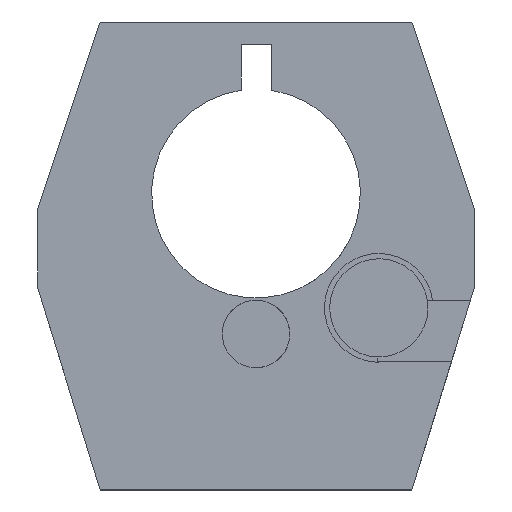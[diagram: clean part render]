
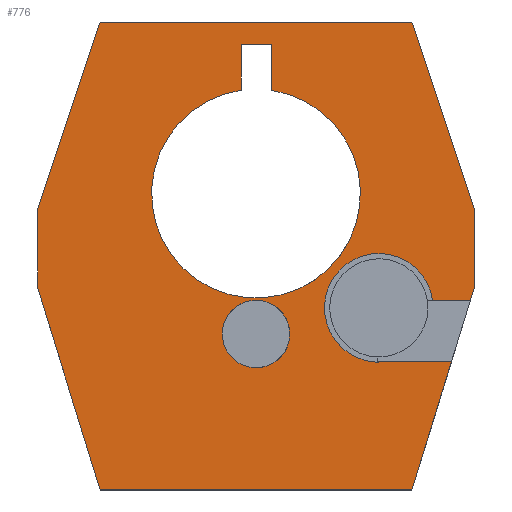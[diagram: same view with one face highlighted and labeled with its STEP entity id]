
A CAD part, front view. The second image highlights one B-rep face of the part: STEP entity #776.
In plain terms, the highlighted planar face has unit normal (0, -1, 0).
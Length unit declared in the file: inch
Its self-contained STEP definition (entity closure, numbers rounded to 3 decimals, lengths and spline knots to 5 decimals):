
#29=FACE_BOUND('',#122,.T.);
#30=FACE_BOUND('',#123,.T.);
#40=CIRCLE('',#836,0.10827);
#41=CIRCLE('',#837,0.10827);
#43=CIRCLE('',#844,0.17421);
#44=CIRCLE('',#846,0.33465);
#77=FACE_OUTER_BOUND('',#121,.T.);
#121=EDGE_LOOP('',(#650,#651,#652,#653,#654,#655,#656,#657,#658,#659,#660,
#661,#662,#663,#664,#665));
#122=EDGE_LOOP('',(#666,#667,#668,#669));
#123=EDGE_LOOP('',(#670,#671));
#162=LINE('',#1124,#253);
#166=LINE('',#1132,#257);
#168=LINE('',#1140,#259);
#174=LINE('',#1152,#265);
#177=LINE('',#1157,#268);
#180=LINE('',#1163,#271);
#184=LINE('',#1172,#275);
#187=LINE('',#1177,#278);
#194=LINE('',#1193,#285);
#203=LINE('',#1226,#294);
#206=LINE('',#1230,#297);
#210=LINE('',#1284,#301);
#212=LINE('',#1289,#303);
#213=LINE('',#1291,#304);
#214=LINE('',#1293,#305);
#215=LINE('',#1295,#306);
#216=LINE('',#1296,#307);
#217=LINE('',#1299,#308);
#253=VECTOR('',#906,0.3937);
#257=VECTOR('',#910,0.3937);
#259=VECTOR('',#918,0.3937);
#265=VECTOR('',#926,0.3937);
#268=VECTOR('',#931,0.3937);
#271=VECTOR('',#936,0.3937);
#275=VECTOR('',#944,0.3937);
#278=VECTOR('',#949,0.3937);
#285=VECTOR('',#962,0.3937);
#294=VECTOR('',#997,0.3937);
#297=VECTOR('',#1002,0.3937);
#301=VECTOR('',#1022,0.3937);
#303=VECTOR('',#1030,0.3937);
#304=VECTOR('',#1031,0.3937);
#305=VECTOR('',#1032,0.3937);
#306=VECTOR('',#1033,0.3937);
#307=VECTOR('',#1034,0.3937);
#308=VECTOR('',#1037,0.3937);
#337=VERTEX_POINT('',#1121);
#338=VERTEX_POINT('',#1123);
#341=VERTEX_POINT('',#1129);
#342=VERTEX_POINT('',#1131);
#345=VERTEX_POINT('',#1139);
#349=VERTEX_POINT('',#1149);
#350=VERTEX_POINT('',#1151);
#351=VERTEX_POINT('',#1155);
#353=VERTEX_POINT('',#1161);
#355=VERTEX_POINT('',#1169);
#356=VERTEX_POINT('',#1171);
#357=VERTEX_POINT('',#1175);
#363=VERTEX_POINT('',#1191);
#373=VERTEX_POINT('',#1223);
#374=VERTEX_POINT('',#1225);
#375=VERTEX_POINT('',#1232);
#376=VERTEX_POINT('',#1233);
#380=VERTEX_POINT('',#1283);
#381=VERTEX_POINT('',#1290);
#382=VERTEX_POINT('',#1292);
#383=VERTEX_POINT('',#1294);
#384=VERTEX_POINT('',#1297);
#416=EDGE_CURVE('',#338,#337,#162,.T.);
#420=EDGE_CURVE('',#342,#341,#166,.T.);
#424=EDGE_CURVE('',#345,#342,#168,.T.);
#430=EDGE_CURVE('',#350,#349,#174,.T.);
#433=EDGE_CURVE('',#349,#351,#177,.T.);
#436=EDGE_CURVE('',#337,#353,#180,.T.);
#440=EDGE_CURVE('',#356,#355,#184,.T.);
#443=EDGE_CURVE('',#355,#357,#187,.T.);
#451=EDGE_CURVE('',#341,#363,#194,.T.);
#466=EDGE_CURVE('',#373,#374,#203,.T.);
#469=EDGE_CURVE('',#345,#373,#206,.T.);
#470=EDGE_CURVE('',#375,#376,#40,.T.);
#471=EDGE_CURVE('',#376,#375,#41,.T.);
#478=EDGE_CURVE('',#380,#338,#210,.T.);
#480=EDGE_CURVE('',#363,#380,#43,.T.);
#481=EDGE_CURVE('',#353,#356,#212,.T.);
#482=EDGE_CURVE('',#357,#381,#213,.T.);
#483=EDGE_CURVE('',#381,#382,#214,.T.);
#484=EDGE_CURVE('',#382,#383,#215,.T.);
#485=EDGE_CURVE('',#383,#374,#216,.T.);
#486=EDGE_CURVE('',#384,#350,#44,.T.);
#487=EDGE_CURVE('',#351,#384,#217,.T.);
#650=ORIENTED_EDGE('',*,*,#451,.T.);
#651=ORIENTED_EDGE('',*,*,#480,.T.);
#652=ORIENTED_EDGE('',*,*,#478,.T.);
#653=ORIENTED_EDGE('',*,*,#416,.T.);
#654=ORIENTED_EDGE('',*,*,#436,.T.);
#655=ORIENTED_EDGE('',*,*,#481,.T.);
#656=ORIENTED_EDGE('',*,*,#440,.T.);
#657=ORIENTED_EDGE('',*,*,#443,.T.);
#658=ORIENTED_EDGE('',*,*,#482,.T.);
#659=ORIENTED_EDGE('',*,*,#483,.T.);
#660=ORIENTED_EDGE('',*,*,#484,.T.);
#661=ORIENTED_EDGE('',*,*,#485,.T.);
#662=ORIENTED_EDGE('',*,*,#466,.F.);
#663=ORIENTED_EDGE('',*,*,#469,.F.);
#664=ORIENTED_EDGE('',*,*,#424,.T.);
#665=ORIENTED_EDGE('',*,*,#420,.T.);
#666=ORIENTED_EDGE('',*,*,#486,.T.);
#667=ORIENTED_EDGE('',*,*,#430,.T.);
#668=ORIENTED_EDGE('',*,*,#433,.T.);
#669=ORIENTED_EDGE('',*,*,#487,.T.);
#670=ORIENTED_EDGE('',*,*,#470,.T.);
#671=ORIENTED_EDGE('',*,*,#471,.T.);
#736=PLANE('',#845);
#776=ADVANCED_FACE('',(#77,#29,#30),#736,.T.);
#836=AXIS2_PLACEMENT_3D('',#1234,#1005,#1006);
#837=AXIS2_PLACEMENT_3D('',#1235,#1007,#1008);
#844=AXIS2_PLACEMENT_3D('',#1287,#1026,#1027);
#845=AXIS2_PLACEMENT_3D('',#1288,#1028,#1029);
#846=AXIS2_PLACEMENT_3D('',#1298,#1035,#1036);
#906=DIRECTION('',(0.294,0.,0.956));
#910=DIRECTION('',(0.294,0.,0.956));
#918=DIRECTION('',(1.,0.,0.));
#926=DIRECTION('',(0.,0.,1.));
#931=DIRECTION('',(1.,0.,0.));
#936=DIRECTION('',(0.,0.,1.));
#944=DIRECTION('',(-1.,0.,0.));
#949=DIRECTION('',(-0.316,0.,-0.949));
#962=DIRECTION('',(-1.,0.,0.));
#997=DIRECTION('',(-1.,0.,0.));
#1002=DIRECTION('',(0.,0.,1.));
#1005=DIRECTION('center_axis',(0.,1.,0.));
#1006=DIRECTION('ref_axis',(1.,0.,0.));
#1007=DIRECTION('center_axis',(0.,1.,0.));
#1008=DIRECTION('ref_axis',(1.,0.,0.));
#1022=DIRECTION('',(1.,0.,0.));
#1026=DIRECTION('center_axis',(0.,1.,0.));
#1027=DIRECTION('ref_axis',(1.,0.,0.));
#1028=DIRECTION('center_axis',(0.,-1.,0.));
#1029=DIRECTION('ref_axis',(0.,0.,-1.));
#1030=DIRECTION('',(-0.316,0.,0.949));
#1031=DIRECTION('',(0.,0.,-1.));
#1032=DIRECTION('',(0.294,0.,-0.956));
#1033=DIRECTION('',(0.294,0.,-0.956));
#1034=DIRECTION('',(0.,0.,1.));
#1035=DIRECTION('center_axis',(0.,1.,0.));
#1036=DIRECTION('ref_axis',(-1.,0.,0.));
#1037=DIRECTION('',(0.,0.,-1.));
#1121=CARTESIAN_POINT('',(0.7,2.56,0.15));
#1123=CARTESIAN_POINT('',(0.68699,2.56,0.10773));
#1124=CARTESIAN_POINT('',(0.5,2.56,-0.5));
#1129=CARTESIAN_POINT('',(0.6264,2.56,-0.08921));
#1131=CARTESIAN_POINT('',(0.5,2.56,-0.5));
#1132=CARTESIAN_POINT('',(0.5,2.56,-0.5));
#1139=CARTESIAN_POINT('',(0.43,2.56,-0.5));
#1140=CARTESIAN_POINT('',(0.43,2.56,-0.5));
#1149=CARTESIAN_POINT('',(-0.0477,2.56,0.92834));
#1151=CARTESIAN_POINT('',(-0.0477,2.56,0.78123));
#1152=CARTESIAN_POINT('',(-0.0477,2.56,0.54213));
#1155=CARTESIAN_POINT('',(0.05072,2.56,0.92834));
#1157=CARTESIAN_POINT('',(-0.22464,2.56,0.92834));
#1161=CARTESIAN_POINT('',(0.7,2.56,0.4));
#1163=CARTESIAN_POINT('',(0.7,2.56,0.15));
#1169=CARTESIAN_POINT('',(-0.5,2.56,1.));
#1171=CARTESIAN_POINT('',(0.5,2.56,1.));
#1172=CARTESIAN_POINT('',(0.5,2.56,1.));
#1175=CARTESIAN_POINT('',(-0.7,2.56,0.4));
#1177=CARTESIAN_POINT('',(-0.7,2.56,0.4));
#1191=CARTESIAN_POINT('',(0.41433,2.56,-0.08921));
#1193=CARTESIAN_POINT('',(0.10264,2.56,-0.08921));
#1223=CARTESIAN_POINT('',(0.43,2.56,-0.49997));
#1225=CARTESIAN_POINT('',(-0.5,2.56,-0.49997));
#1226=CARTESIAN_POINT('',(-0.14192,2.56,-0.49997));
#1230=CARTESIAN_POINT('',(0.43,2.56,-0.5));
#1232=CARTESIAN_POINT('',(-0.05174,2.56,0.0951));
#1233=CARTESIAN_POINT('',(-0.10827,2.56,0.));
#1234=CARTESIAN_POINT('Origin',(0.,2.56,0.));
#1235=CARTESIAN_POINT('Origin',(0.,2.56,0.));
#1283=CARTESIAN_POINT('',(0.56626,2.56,0.10773));
#1284=CARTESIAN_POINT('',(0.03313,2.56,0.10773));
#1287=CARTESIAN_POINT('Origin',(0.3937,2.56,0.08378));
#1288=CARTESIAN_POINT('Origin',(-0.5,2.56,0.29994));
#1289=CARTESIAN_POINT('',(0.7,2.56,0.4));
#1290=CARTESIAN_POINT('',(-0.7,2.56,0.15));
#1291=CARTESIAN_POINT('',(-0.7,2.56,0.4));
#1292=CARTESIAN_POINT('',(-0.60447,2.56,-0.16048));
#1293=CARTESIAN_POINT('',(-0.7,2.56,0.15));
#1294=CARTESIAN_POINT('',(-0.5,2.56,-0.5));
#1295=CARTESIAN_POINT('',(-0.60447,2.56,-0.16048));
#1296=CARTESIAN_POINT('',(-0.5,2.56,-0.5));
#1297=CARTESIAN_POINT('',(0.05072,2.56,0.78078));
#1298=CARTESIAN_POINT('Origin',(0.,2.56,0.45));
#1299=CARTESIAN_POINT('',(0.05072,2.56,0.46835));
